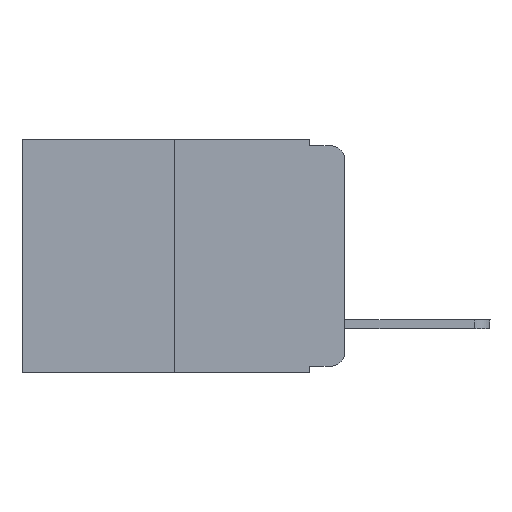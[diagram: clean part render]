
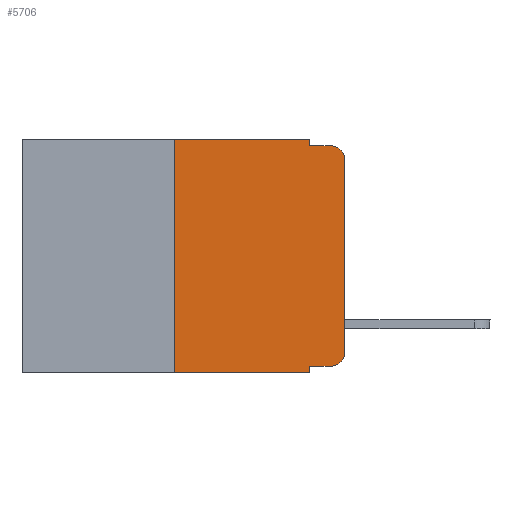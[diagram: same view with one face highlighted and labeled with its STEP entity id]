
A CAD part, left-side view. The second image highlights one B-rep face of the part: STEP entity #5706.
In plain terms, the highlighted planar face has unit normal (-1, 0, 0).
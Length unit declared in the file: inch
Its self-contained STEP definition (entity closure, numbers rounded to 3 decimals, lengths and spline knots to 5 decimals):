
#94 = LINE ( 'NONE', #4943, #1023 ) ;
#188 = VECTOR ( 'NONE', #3097, 39.37008 ) ;
#249 = DIRECTION ( 'NONE',  ( 0., 0., -1. ) ) ;
#331 = VECTOR ( 'NONE', #4192, 39.37008 ) ;
#370 = VERTEX_POINT ( 'NONE', #9978 ) ;
#767 = CARTESIAN_POINT ( 'NONE',  ( 0., 0.02, -0.313 ) ) ;
#789 = FACE_OUTER_BOUND ( 'NONE', #9921, .T. ) ;
#870 = LINE ( 'NONE', #1303, #7321 ) ;
#972 = LINE ( 'NONE', #4067, #188 ) ;
#1023 = VECTOR ( 'NONE', #5744, 39.37008 ) ;
#1221 = VERTEX_POINT ( 'NONE', #7264 ) ;
#1303 = CARTESIAN_POINT ( 'NONE',  ( 0., 0.051, -0.333 ) ) ;
#1438 = ORIENTED_EDGE ( 'NONE', *, *, #8669, .F. ) ;
#1609 = DIRECTION ( 'NONE',  ( 0., 0., -1. ) ) ;
#1634 = VECTOR ( 'NONE', #6364, 39.37008 ) ;
#1740 = EDGE_CURVE ( 'NONE', #370, #4048, #972, .T. ) ;
#1753 = EDGE_CURVE ( 'NONE', #6822, #5496, #7930, .T. ) ;
#1957 = CARTESIAN_POINT ( 'NONE',  ( 0., 0.25, 0. ) ) ;
#2012 = ORIENTED_EDGE ( 'NONE', *, *, #9064, .T. ) ;
#2066 = LINE ( 'NONE', #2189, #8150 ) ;
#2189 = CARTESIAN_POINT ( 'NONE',  ( 0., 0.473, 0. ) ) ;
#2481 = VERTEX_POINT ( 'NONE', #2971 ) ;
#2923 = LINE ( 'NONE', #7710, #1634 ) ;
#2971 = CARTESIAN_POINT ( 'NONE',  ( 0., 0.02, -0.01 ) ) ;
#3097 = DIRECTION ( 'NONE',  ( 0., -1., 0. ) ) ;
#3101 = VERTEX_POINT ( 'NONE', #5850 ) ;
#3308 = ORIENTED_EDGE ( 'NONE', *, *, #7733, .T. ) ;
#3379 = VERTEX_POINT ( 'NONE', #6244 ) ;
#3700 = DIRECTION ( 'NONE',  ( 0., 0., 1. ) ) ;
#3885 = DIRECTION ( 'NONE',  ( 0., -1., 0. ) ) ;
#3924 = LINE ( 'NONE', #10084, #4834 ) ;
#3931 = LINE ( 'NONE', #8313, #331 ) ;
#4048 = VERTEX_POINT ( 'NONE', #7996 ) ;
#4067 = CARTESIAN_POINT ( 'NONE',  ( 0., 0.473, -0.343 ) ) ;
#4102 = VERTEX_POINT ( 'NONE', #8844 ) ;
#4124 = CARTESIAN_POINT ( 'NONE',  ( 0., 0.02, -0.333 ) ) ;
#4192 = DIRECTION ( 'NONE',  ( 0., 0., -1. ) ) ;
#4392 = DIRECTION ( 'NONE',  ( -1., 0., 0. ) ) ;
#4456 = ORIENTED_EDGE ( 'NONE', *, *, #9849, .F. ) ;
#4834 = VECTOR ( 'NONE', #10113, 39.37008 ) ;
#4943 = CARTESIAN_POINT ( 'NONE',  ( 0., 0., 0. ) ) ;
#4983 = AXIS2_PLACEMENT_3D ( 'NONE', #5695, #8945, #1609 ) ;
#5087 = AXIS2_PLACEMENT_3D ( 'NONE', #9451, #10215, #249 ) ;
#5202 = PLANE ( 'NONE',  #5087 ) ;
#5324 = EDGE_CURVE ( 'NONE', #4102, #1221, #2066, .T. ) ;
#5496 = VERTEX_POINT ( 'NONE', #8415 ) ;
#5504 = CIRCLE ( 'NONE', #4983, 0.02 ) ;
#5695 = CARTESIAN_POINT ( 'NONE',  ( 0., 0.02, -0.03 ) ) ;
#5706 = ADVANCED_FACE ( 'NONE', ( #789 ), #5202, .F. ) ;
#5744 = DIRECTION ( 'NONE',  ( 0., 0., 1. ) ) ;
#5847 = LINE ( 'NONE', #1957, #8715 ) ;
#5850 = CARTESIAN_POINT ( 'NONE',  ( 0., 0.051, -0.01 ) ) ;
#6244 = CARTESIAN_POINT ( 'NONE',  ( 0., 0., -0.03 ) ) ;
#6364 = DIRECTION ( 'NONE',  ( 0., -1., 0. ) ) ;
#6501 = CARTESIAN_POINT ( 'NONE',  ( 0., 0.051, -0.333 ) ) ;
#6739 = VERTEX_POINT ( 'NONE', #6501 ) ;
#6822 = VERTEX_POINT ( 'NONE', #4124 ) ;
#6888 = ORIENTED_EDGE ( 'NONE', *, *, #8289, .F. ) ;
#7118 = ORIENTED_EDGE ( 'NONE', *, *, #10611, .F. ) ;
#7257 = EDGE_CURVE ( 'NONE', #5496, #3379, #94, .T. ) ;
#7264 = CARTESIAN_POINT ( 'NONE',  ( 0., 0.051, 0. ) ) ;
#7321 = VECTOR ( 'NONE', #8787, 39.37008 ) ;
#7710 = CARTESIAN_POINT ( 'NONE',  ( 0., 0.051, -0.01 ) ) ;
#7733 = EDGE_CURVE ( 'NONE', #6739, #6822, #870, .T. ) ;
#7930 = CIRCLE ( 'NONE', #9569, 0.02 ) ;
#7996 = CARTESIAN_POINT ( 'NONE',  ( 0., 0.051, -0.343 ) ) ;
#8150 = VECTOR ( 'NONE', #3885, 39.37008 ) ;
#8289 = EDGE_CURVE ( 'NONE', #3101, #2481, #2923, .T. ) ;
#8313 = CARTESIAN_POINT ( 'NONE',  ( 0., 0.051, 0. ) ) ;
#8415 = CARTESIAN_POINT ( 'NONE',  ( 0., 0., -0.313 ) ) ;
#8669 = EDGE_CURVE ( 'NONE', #1221, #3101, #3931, .T. ) ;
#8715 = VECTOR ( 'NONE', #3700, 39.37008 ) ;
#8787 = DIRECTION ( 'NONE',  ( 0., -1., 0. ) ) ;
#8844 = CARTESIAN_POINT ( 'NONE',  ( 0., 0.25, 0. ) ) ;
#8853 = DIRECTION ( 'NONE',  ( 0., 0., -1. ) ) ;
#8945 = DIRECTION ( 'NONE',  ( -1., 0., 0. ) ) ;
#9031 = ORIENTED_EDGE ( 'NONE', *, *, #7257, .T. ) ;
#9064 = EDGE_CURVE ( 'NONE', #3379, #2481, #5504, .T. ) ;
#9451 = CARTESIAN_POINT ( 'NONE',  ( 0., 0.473, 0. ) ) ;
#9569 = AXIS2_PLACEMENT_3D ( 'NONE', #767, #4392, #8853 ) ;
#9643 = ORIENTED_EDGE ( 'NONE', *, *, #5324, .F. ) ;
#9652 = ORIENTED_EDGE ( 'NONE', *, *, #1740, .T. ) ;
#9849 = EDGE_CURVE ( 'NONE', #6739, #4048, #3924, .T. ) ;
#9921 = EDGE_LOOP ( 'NONE', ( #9031, #2012, #6888, #1438, #9643, #7118, #9652, #4456, #3308, #10028 ) ) ;
#9978 = CARTESIAN_POINT ( 'NONE',  ( 0., 0.25, -0.343 ) ) ;
#10028 = ORIENTED_EDGE ( 'NONE', *, *, #1753, .T. ) ;
#10084 = CARTESIAN_POINT ( 'NONE',  ( 0., 0.051, 0. ) ) ;
#10113 = DIRECTION ( 'NONE',  ( 0., 0., -1. ) ) ;
#10215 = DIRECTION ( 'NONE',  ( 1., 0., 0. ) ) ;
#10611 = EDGE_CURVE ( 'NONE', #370, #4102, #5847, .T. ) ;
